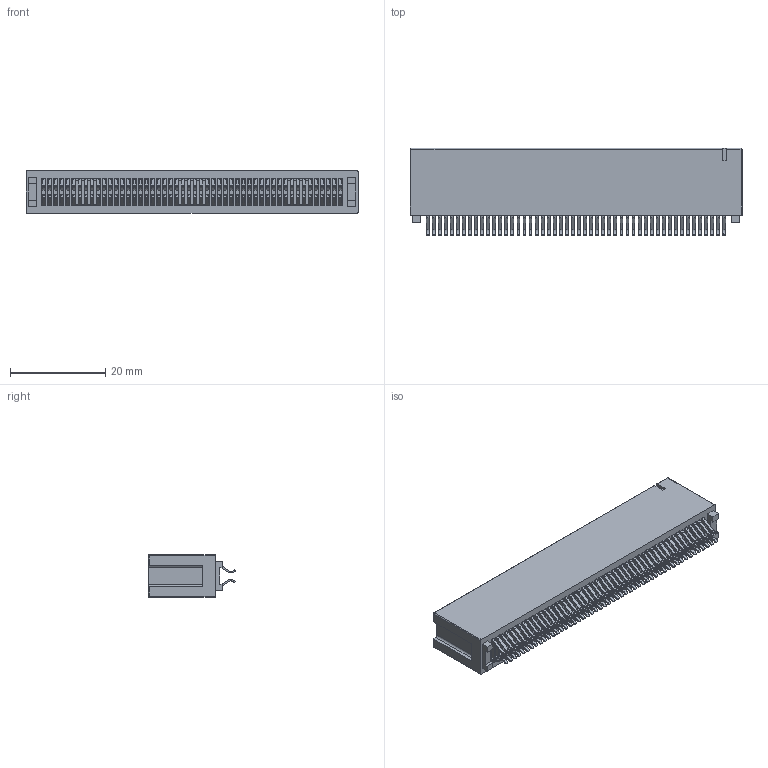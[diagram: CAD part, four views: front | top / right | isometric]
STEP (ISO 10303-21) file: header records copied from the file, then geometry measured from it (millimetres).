
FILE_DESCRIPTION (( 'STEP AP203' ), '1' );
FILE_NAME ('302-100-656-201.STEP', '2024-04-06T14:35:26', ( '' ), ( '' ), 'SwSTEP 2.0', 'SolidWorks 2023', '' );
FILE_SCHEMA (( 'CONFIG_CONTROL_DESIGN' ));
Length unit declared in the file: millimetre
Products named in the file (3): 302-100-656-201; HSG_Vertical HSG; Contact_302-290-X56
Assembly tree (101 placements, depth 2):
  302-100-656-201
    HSG_Vertical HSG
    Contact_302-290-X56  x100
Bounding box: 69.6 x 18.3 x 8.88 mm (x, y, z)
Volume: 5341.4 mm3; surface area: 15222.8 mm2
Topology: 101 solids, 101 shells, 4816 faces, 14368 edges, 9504 vertices
Faces by surface type: plane 3199, cylinder 1613, sphere 4
Entity records: 37995 total; most frequent: ORIENTED_EDGE 6552, CARTESIAN_POINT 6434, DIRECTION 5246, EDGE_CURVE 3276, LINE 3218, VECTOR 3218, VERTEX_POINT 2178, AXIS2_PLACEMENT_3D 1014
